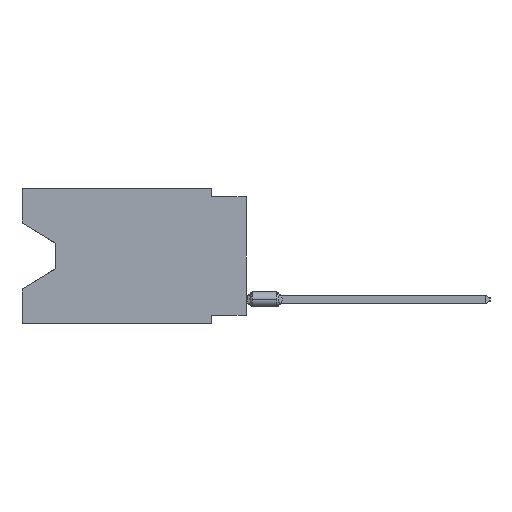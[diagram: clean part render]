
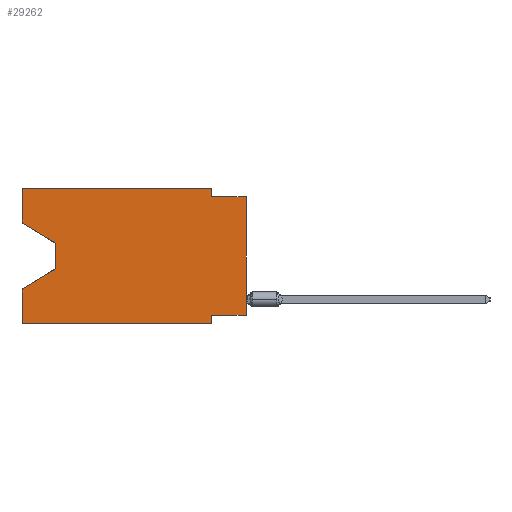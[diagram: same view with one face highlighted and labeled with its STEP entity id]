
A CAD part, left-side view. The second image highlights one B-rep face of the part: STEP entity #29262.
In plain terms, the highlighted planar face has unit normal (-1, 0, 0).
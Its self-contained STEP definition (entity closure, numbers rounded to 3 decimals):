
#154 = CARTESIAN_POINT ( 'NONE',  ( 0., 2.54, 0. ) ) ;
#312 = VECTOR ( 'NONE', #42375, 1000. ) ;
#970 = VERTEX_POINT ( 'NONE', #51381 ) ;
#1523 = LINE ( 'NONE', #28579, #312 ) ;
#3229 = CARTESIAN_POINT ( 'NONE',  ( 0., 16.383, 0. ) ) ;
#3642 = LINE ( 'NONE', #4262, #45836 ) ;
#4262 = CARTESIAN_POINT ( 'NONE',  ( 0., 16.383, 0. ) ) ;
#4409 = DIRECTION ( 'NONE',  ( 0., -0.855, -0.519 ) ) ;
#4577 = CARTESIAN_POINT ( 'NONE',  ( 0., 2.54, -9.271 ) ) ;
#4900 = CARTESIAN_POINT ( 'NONE',  ( 0., 16.383, -9.906 ) ) ;
#5330 = VERTEX_POINT ( 'NONE', #35637 ) ;
#5342 = DIRECTION ( 'NONE',  ( 0., 0., 1. ) ) ;
#6262 = CARTESIAN_POINT ( 'NONE',  ( 0., 13.97, -5.893 ) ) ;
#6285 = EDGE_CURVE ( 'NONE', #17292, #23190, #3642, .T. ) ;
#8553 = FACE_OUTER_BOUND ( 'NONE', #45360, .T. ) ;
#8868 = VECTOR ( 'NONE', #5342, 1000. ) ;
#8896 = CARTESIAN_POINT ( 'NONE',  ( 0., 13.97, -5.893 ) ) ;
#9292 = VERTEX_POINT ( 'NONE', #51952 ) ;
#9423 = CARTESIAN_POINT ( 'NONE',  ( 0., 2.54, 0. ) ) ;
#9495 = CARTESIAN_POINT ( 'NONE',  ( 0., 16.383, -2.546 ) ) ;
#10124 = CARTESIAN_POINT ( 'NONE',  ( 0., 16.383, 0. ) ) ;
#10970 = EDGE_CURVE ( 'NONE', #17292, #58318, #54551, .T. ) ;
#10998 = EDGE_CURVE ( 'NONE', #26068, #9292, #50058, .T. ) ;
#11132 = EDGE_CURVE ( 'NONE', #5330, #970, #29305, .T. ) ;
#11972 = ORIENTED_EDGE ( 'NONE', *, *, #6285, .F. ) ;
#12169 = ORIENTED_EDGE ( 'NONE', *, *, #11132, .T. ) ;
#12289 = VECTOR ( 'NONE', #49384, 1000. ) ;
#13040 = LINE ( 'NONE', #9423, #12289 ) ;
#13191 = VECTOR ( 'NONE', #29532, 1000. ) ;
#13702 = LINE ( 'NONE', #32308, #28019 ) ;
#14631 = ORIENTED_EDGE ( 'NONE', *, *, #34925, .F. ) ;
#14855 = ORIENTED_EDGE ( 'NONE', *, *, #45858, .T. ) ;
#16055 = CARTESIAN_POINT ( 'NONE',  ( 0., 0., -0.635 ) ) ;
#17002 = LINE ( 'NONE', #56217, #20038 ) ;
#17004 = VERTEX_POINT ( 'NONE', #18796 ) ;
#17038 = EDGE_CURVE ( 'NONE', #17004, #970, #24775, .T. ) ;
#17292 = VERTEX_POINT ( 'NONE', #57776 ) ;
#18107 = VERTEX_POINT ( 'NONE', #4900 ) ;
#18796 = CARTESIAN_POINT ( 'NONE',  ( 0., 2.54, -0.635 ) ) ;
#19525 = CARTESIAN_POINT ( 'NONE',  ( 0., 2.54, -9.906 ) ) ;
#19616 = EDGE_CURVE ( 'NONE', #52189, #45033, #13702, .T. ) ;
#20009 = EDGE_CURVE ( 'NONE', #18107, #9292, #42567, .T. ) ;
#20038 = VECTOR ( 'NONE', #29796, 1000. ) ;
#20071 = ORIENTED_EDGE ( 'NONE', *, *, #51222, .F. ) ;
#21773 = DIRECTION ( 'NONE',  ( 1., 0., 0. ) ) ;
#21966 = DIRECTION ( 'NONE',  ( 0., 0., 1. ) ) ;
#21992 = VECTOR ( 'NONE', #41062, 1000. ) ;
#23190 = VERTEX_POINT ( 'NONE', #10124 ) ;
#23335 = ORIENTED_EDGE ( 'NONE', *, *, #19616, .F. ) ;
#24775 = LINE ( 'NONE', #16055, #41386 ) ;
#24837 = CARTESIAN_POINT ( 'NONE',  ( 0., 16.383, 0. ) ) ;
#25045 = ORIENTED_EDGE ( 'NONE', *, *, #20009, .F. ) ;
#26068 = VERTEX_POINT ( 'NONE', #6262 ) ;
#26544 = VECTOR ( 'NONE', #4409, 1000. ) ;
#27248 = DIRECTION ( 'NONE',  ( 0., 0.855, -0.519 ) ) ;
#27554 = VERTEX_POINT ( 'NONE', #154 ) ;
#27833 = CARTESIAN_POINT ( 'NONE',  ( 0., 13.97, -4.013 ) ) ;
#28019 = VECTOR ( 'NONE', #31424, 1000. ) ;
#28083 = ORIENTED_EDGE ( 'NONE', *, *, #10998, .T. ) ;
#28089 = ORIENTED_EDGE ( 'NONE', *, *, #10970, .T. ) ;
#28579 = CARTESIAN_POINT ( 'NONE',  ( 0., 0., -9.271 ) ) ;
#29262 = ADVANCED_FACE ( 'NONE', ( #8553 ), #40709, .F. ) ;
#29305 = LINE ( 'NONE', #37424, #38028 ) ;
#29532 = DIRECTION ( 'NONE',  ( 0., 0., -1. ) ) ;
#29796 = DIRECTION ( 'NONE',  ( 0., -1., 0. ) ) ;
#30857 = LINE ( 'NONE', #3229, #21992 ) ;
#31424 = DIRECTION ( 'NONE',  ( 0., 0., -1. ) ) ;
#32308 = CARTESIAN_POINT ( 'NONE',  ( 0., 2.54, -9.906 ) ) ;
#33221 = DIRECTION ( 'NONE',  ( 0., 0., 1. ) ) ;
#34925 = EDGE_CURVE ( 'NONE', #27554, #17004, #13040, .T. ) ;
#35004 = ORIENTED_EDGE ( 'NONE', *, *, #17038, .F. ) ;
#35637 = CARTESIAN_POINT ( 'NONE',  ( 0., 0., -9.271 ) ) ;
#37424 = CARTESIAN_POINT ( 'NONE',  ( 0., 0., 0. ) ) ;
#38028 = VECTOR ( 'NONE', #33221, 1000. ) ;
#40709 = PLANE ( 'NONE',  #41583 ) ;
#41062 = DIRECTION ( 'NONE',  ( 0., -1., 0. ) ) ;
#41386 = VECTOR ( 'NONE', #56584, 1000. ) ;
#41583 = AXIS2_PLACEMENT_3D ( 'NONE', #44602, #21773, #49415 ) ;
#41622 = EDGE_CURVE ( 'NONE', #58318, #26068, #48438, .T. ) ;
#42375 = DIRECTION ( 'NONE',  ( 0., 1., 0. ) ) ;
#42567 = LINE ( 'NONE', #24837, #8868 ) ;
#43054 = ORIENTED_EDGE ( 'NONE', *, *, #41622, .T. ) ;
#44602 = CARTESIAN_POINT ( 'NONE',  ( 0., 16.383, 0. ) ) ;
#45033 = VERTEX_POINT ( 'NONE', #19525 ) ;
#45360 = EDGE_LOOP ( 'NONE', ( #28089, #43054, #28083, #25045, #14855, #23335, #52746, #12169, #35004, #14631, #20071, #11972 ) ) ;
#45836 = VECTOR ( 'NONE', #21966, 1000. ) ;
#45858 = EDGE_CURVE ( 'NONE', #18107, #45033, #17002, .T. ) ;
#48438 = LINE ( 'NONE', #52353, #13191 ) ;
#49384 = DIRECTION ( 'NONE',  ( 0., 0., -1. ) ) ;
#49415 = DIRECTION ( 'NONE',  ( 0., 0., -1. ) ) ;
#50058 = LINE ( 'NONE', #8896, #54307 ) ;
#50304 = EDGE_CURVE ( 'NONE', #5330, #52189, #1523, .T. ) ;
#51222 = EDGE_CURVE ( 'NONE', #23190, #27554, #30857, .T. ) ;
#51381 = CARTESIAN_POINT ( 'NONE',  ( 0., 0., -0.635 ) ) ;
#51952 = CARTESIAN_POINT ( 'NONE',  ( 0., 16.383, -7.36 ) ) ;
#52189 = VERTEX_POINT ( 'NONE', #4577 ) ;
#52353 = CARTESIAN_POINT ( 'NONE',  ( 0., 13.97, -4.013 ) ) ;
#52746 = ORIENTED_EDGE ( 'NONE', *, *, #50304, .F. ) ;
#54307 = VECTOR ( 'NONE', #27248, 1000. ) ;
#54551 = LINE ( 'NONE', #9495, #26544 ) ;
#56217 = CARTESIAN_POINT ( 'NONE',  ( 0., 16.383, -9.906 ) ) ;
#56584 = DIRECTION ( 'NONE',  ( 0., -1., 0. ) ) ;
#57776 = CARTESIAN_POINT ( 'NONE',  ( 0., 16.383, -2.546 ) ) ;
#58318 = VERTEX_POINT ( 'NONE', #27833 ) ;
